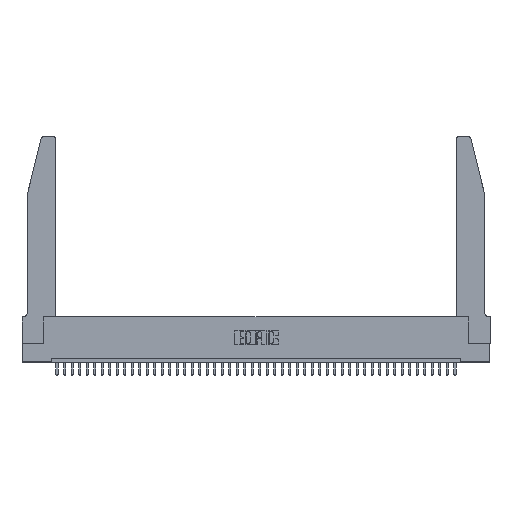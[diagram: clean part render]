
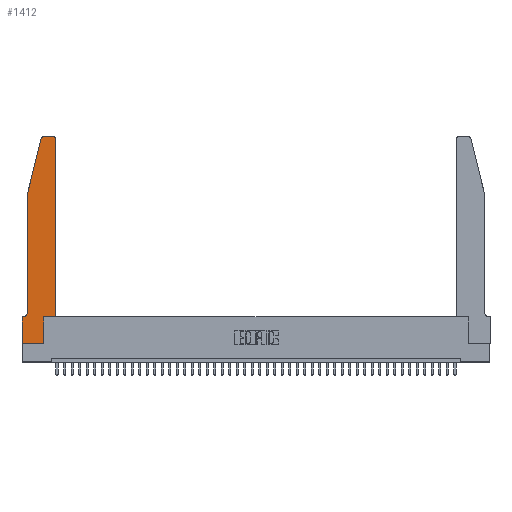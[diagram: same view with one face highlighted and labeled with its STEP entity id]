
A CAD part, top view. The second image highlights one B-rep face of the part: STEP entity #1412.
In plain terms, the highlighted planar face has unit normal (0, 0, 1).
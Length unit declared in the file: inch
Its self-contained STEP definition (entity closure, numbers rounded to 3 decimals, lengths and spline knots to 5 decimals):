
#210 = CARTESIAN_POINT ( 'NONE',  ( 0.4205, 2.72, 0.37 ) ) ;
#258 = CARTESIAN_POINT ( 'NONE',  ( 0.0755, 2., 0.37 ) ) ;
#731 = EDGE_CURVE ( 'NONE', #29556, #43133, #3555, .T. ) ;
#1345 = CARTESIAN_POINT ( 'NONE',  ( 0.4205, 2.75, 0.37 ) ) ;
#1412 = ADVANCED_FACE ( 'NONE', ( #9259 ), #25542, .T. ) ;
#1779 = CARTESIAN_POINT ( 'NONE',  ( 0.0055, 0.35, 0.37 ) ) ;
#1851 = VECTOR ( 'NONE', #7480, 39.37008 ) ;
#1991 = CARTESIAN_POINT ( 'NONE',  ( 0.0755, 2., 0.37 ) ) ;
#2315 = AXIS2_PLACEMENT_3D ( 'NONE', #35466, #41825, #25074 ) ;
#2583 = EDGE_CURVE ( 'NONE', #6032, #38369, #41634, .T. ) ;
#2813 = DIRECTION ( 'NONE',  ( 0., -1., 0. ) ) ;
#2998 = EDGE_CURVE ( 'NONE', #8180, #35416, #35467, .T. ) ;
#3555 = LINE ( 'NONE', #36514, #37060 ) ;
#3847 = ORIENTED_EDGE ( 'NONE', *, *, #731, .T. ) ;
#4953 = ORIENTED_EDGE ( 'NONE', *, *, #22148, .T. ) ;
#5146 = DIRECTION ( 'NONE',  ( 1., 0., 0. ) ) ;
#5342 = DIRECTION ( 'NONE',  ( 0., -1., 0. ) ) ;
#6032 = VERTEX_POINT ( 'NONE', #19508 ) ;
#6077 = EDGE_CURVE ( 'NONE', #35416, #6032, #23540, .T. ) ;
#6538 = CARTESIAN_POINT ( 'NONE',  ( 0.2865, 0.35, 0.37 ) ) ;
#6598 = DIRECTION ( 'NONE',  ( 1., 0., 0. ) ) ;
#6721 = DIRECTION ( 'NONE',  ( 0., 1., 0. ) ) ;
#6770 = EDGE_CURVE ( 'NONE', #27404, #28813, #24537, .T. ) ;
#6845 = EDGE_CURVE ( 'NONE', #28813, #11604, #19181, .T. ) ;
#7480 = DIRECTION ( 'NONE',  ( -0.239, -0.971, 0. ) ) ;
#7718 = CARTESIAN_POINT ( 'NONE',  ( 0., 0., 0.37 ) ) ;
#7931 = AXIS2_PLACEMENT_3D ( 'NONE', #43113, #22819, #5146 ) ;
#8180 = VERTEX_POINT ( 'NONE', #1345 ) ;
#8314 = VECTOR ( 'NONE', #23439, 39.37008 ) ;
#9093 = CARTESIAN_POINT ( 'NONE',  ( 0.0755, 2., 0.37 ) ) ;
#9259 = FACE_OUTER_BOUND ( 'NONE', #12731, .T. ) ;
#10569 = CARTESIAN_POINT ( 'NONE',  ( 0.0055, 0.42, 0.37 ) ) ;
#10839 = EDGE_CURVE ( 'NONE', #43133, #22242, #43390, .T. ) ;
#11604 = VERTEX_POINT ( 'NONE', #39434 ) ;
#12600 = CARTESIAN_POINT ( 'NONE',  ( 0., 0., 0.37 ) ) ;
#12731 = EDGE_LOOP ( 'NONE', ( #30282, #30498, #34340, #4953, #22268, #33952, #18890, #3847, #22540, #28009, #26612, #14523 ) ) ;
#13861 = DIRECTION ( 'NONE',  ( 1., 0., 0. ) ) ;
#14523 = ORIENTED_EDGE ( 'NONE', *, *, #39956, .T. ) ;
#15606 = VECTOR ( 'NONE', #5342, 39.37008 ) ;
#16302 = VECTOR ( 'NONE', #30183, 39.37008 ) ;
#18070 = DIRECTION ( 'NONE',  ( -1., 0., 0. ) ) ;
#18890 = ORIENTED_EDGE ( 'NONE', *, *, #43189, .T. ) ;
#19005 = VECTOR ( 'NONE', #2813, 39.37008 ) ;
#19115 = CARTESIAN_POINT ( 'NONE',  ( 0.2865, 0.35, 0.37 ) ) ;
#19181 = LINE ( 'NONE', #32113, #22416 ) ;
#19470 = CIRCLE ( 'NONE', #28465, 0.03 ) ;
#19508 = CARTESIAN_POINT ( 'NONE',  ( 0.25487, 2.72718, 0.37 ) ) ;
#20075 = LINE ( 'NONE', #9093, #19005 ) ;
#20364 = LINE ( 'NONE', #12600, #15606 ) ;
#21320 = CARTESIAN_POINT ( 'NONE',  ( 0.4505, 0.35, 0.37 ) ) ;
#21694 = DIRECTION ( 'NONE',  ( 0., 0., -1. ) ) ;
#22148 = EDGE_CURVE ( 'NONE', #38369, #27404, #20075, .T. ) ;
#22160 = EDGE_CURVE ( 'NONE', #31643, #26649, #22187, .T. ) ;
#22187 = LINE ( 'NONE', #36942, #28652 ) ;
#22242 = VERTEX_POINT ( 'NONE', #19115 ) ;
#22268 = ORIENTED_EDGE ( 'NONE', *, *, #6770, .T. ) ;
#22416 = VECTOR ( 'NONE', #18070, 39.37008 ) ;
#22540 = ORIENTED_EDGE ( 'NONE', *, *, #10839, .T. ) ;
#22819 = DIRECTION ( 'NONE',  ( 0., 0., 1. ) ) ;
#23439 = DIRECTION ( 'NONE',  ( -1., 0., 0. ) ) ;
#23540 = CIRCLE ( 'NONE', #7931, 0.03 ) ;
#23553 = DIRECTION ( 'NONE',  ( 0., 0., 1. ) ) ;
#24537 = CIRCLE ( 'NONE', #26851, 0.07 ) ;
#25074 = DIRECTION ( 'NONE',  ( 1., 0., 0. ) ) ;
#25542 = PLANE ( 'NONE',  #2315 ) ;
#26612 = ORIENTED_EDGE ( 'NONE', *, *, #22160, .T. ) ;
#26649 = VERTEX_POINT ( 'NONE', #31125 ) ;
#26851 = AXIS2_PLACEMENT_3D ( 'NONE', #10569, #21694, #30201 ) ;
#27404 = VERTEX_POINT ( 'NONE', #40709 ) ;
#27899 = CARTESIAN_POINT ( 'NONE',  ( 0.2865, 0., 0.37 ) ) ;
#28009 = ORIENTED_EDGE ( 'NONE', *, *, #36467, .T. ) ;
#28066 = DIRECTION ( 'NONE',  ( 1., 0., 0. ) ) ;
#28465 = AXIS2_PLACEMENT_3D ( 'NONE', #210, #23553, #6598 ) ;
#28610 = CARTESIAN_POINT ( 'NONE',  ( 0.284, 2.75, 0.37 ) ) ;
#28652 = VECTOR ( 'NONE', #6721, 39.37008 ) ;
#28695 = CARTESIAN_POINT ( 'NONE',  ( 0.4505, 0.35, 0.37 ) ) ;
#28813 = VERTEX_POINT ( 'NONE', #1779 ) ;
#29556 = VERTEX_POINT ( 'NONE', #7718 ) ;
#30183 = DIRECTION ( 'NONE',  ( 0., 1., 0. ) ) ;
#30201 = DIRECTION ( 'NONE',  ( -1., 0., 0. ) ) ;
#30282 = ORIENTED_EDGE ( 'NONE', *, *, #2998, .T. ) ;
#30405 = LINE ( 'NONE', #21320, #37326 ) ;
#30498 = ORIENTED_EDGE ( 'NONE', *, *, #6077, .T. ) ;
#31125 = CARTESIAN_POINT ( 'NONE',  ( 0.4505, 2.72, 0.37 ) ) ;
#31643 = VERTEX_POINT ( 'NONE', #28695 ) ;
#32113 = CARTESIAN_POINT ( 'NONE',  ( 0.0755, 0.35, 0.37 ) ) ;
#33952 = ORIENTED_EDGE ( 'NONE', *, *, #6845, .T. ) ;
#34340 = ORIENTED_EDGE ( 'NONE', *, *, #2583, .T. ) ;
#35416 = VERTEX_POINT ( 'NONE', #28610 ) ;
#35466 = CARTESIAN_POINT ( 'NONE',  ( 0., 0.35, 0.37 ) ) ;
#35467 = LINE ( 'NONE', #37130, #8314 ) ;
#36467 = EDGE_CURVE ( 'NONE', #22242, #31643, #30405, .T. ) ;
#36514 = CARTESIAN_POINT ( 'NONE',  ( 0., 0., 0.37 ) ) ;
#36942 = CARTESIAN_POINT ( 'NONE',  ( 0.4505, 0.35, 0.37 ) ) ;
#37060 = VECTOR ( 'NONE', #13861, 39.37008 ) ;
#37130 = CARTESIAN_POINT ( 'NONE',  ( 0.2605, 2.75, 0.37 ) ) ;
#37326 = VECTOR ( 'NONE', #28066, 39.37008 ) ;
#38369 = VERTEX_POINT ( 'NONE', #1991 ) ;
#39434 = CARTESIAN_POINT ( 'NONE',  ( 0., 0.35, 0.37 ) ) ;
#39956 = EDGE_CURVE ( 'NONE', #26649, #8180, #19470, .T. ) ;
#40709 = CARTESIAN_POINT ( 'NONE',  ( 0.0755, 0.42, 0.37 ) ) ;
#41634 = LINE ( 'NONE', #258, #1851 ) ;
#41825 = DIRECTION ( 'NONE',  ( 0., 0., 1. ) ) ;
#43113 = CARTESIAN_POINT ( 'NONE',  ( 0.284, 2.72, 0.37 ) ) ;
#43133 = VERTEX_POINT ( 'NONE', #27899 ) ;
#43189 = EDGE_CURVE ( 'NONE', #11604, #29556, #20364, .T. ) ;
#43390 = LINE ( 'NONE', #6538, #16302 ) ;
